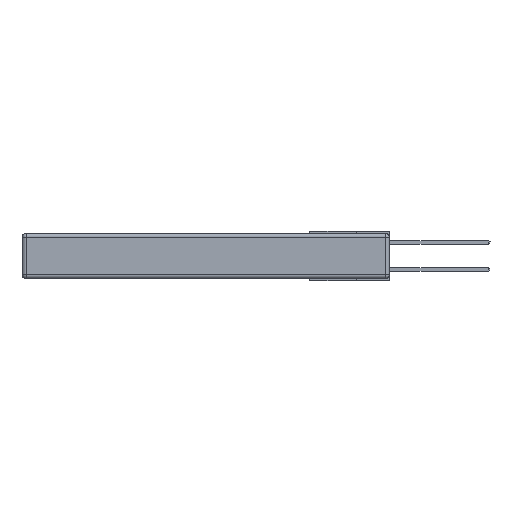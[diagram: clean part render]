
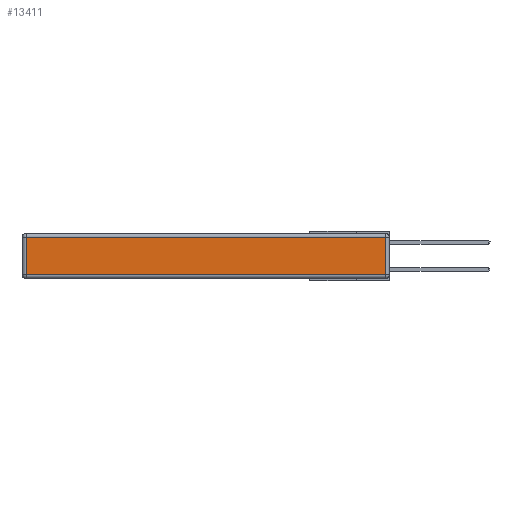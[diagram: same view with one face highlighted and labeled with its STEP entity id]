
A CAD part, left-side view. The second image highlights one B-rep face of the part: STEP entity #13411.
In plain terms, the highlighted planar face has unit normal (-1, 0, 0).
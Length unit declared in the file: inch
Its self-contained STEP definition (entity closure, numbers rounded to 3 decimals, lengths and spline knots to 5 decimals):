
#1149 = VERTEX_POINT ( 'NONE', #26603 ) ;
#1266 = CARTESIAN_POINT ( 'NONE',  ( 0., 2.75, -0.03 ) ) ;
#1762 = EDGE_LOOP ( 'NONE', ( #14225, #14690, #22841, #14623 ) ) ;
#2381 = VECTOR ( 'NONE', #23306, 39.37008 ) ;
#2400 = EDGE_CURVE ( 'NONE', #9237, #16036, #15914, .T. ) ;
#2862 = CARTESIAN_POINT ( 'NONE',  ( 0., 0.03, -0.343 ) ) ;
#3988 = EDGE_CURVE ( 'NONE', #16036, #24793, #28977, .T. ) ;
#4925 = DIRECTION ( 'NONE',  ( 0., 0., 1. ) ) ;
#7043 = PLANE ( 'NONE',  #23696 ) ;
#7703 = DIRECTION ( 'NONE',  ( 0., 1., 0. ) ) ;
#8486 = LINE ( 'NONE', #2862, #2381 ) ;
#9237 = VERTEX_POINT ( 'NONE', #14497 ) ;
#10323 = EDGE_CURVE ( 'NONE', #1149, #9237, #8486, .T. ) ;
#11277 = VECTOR ( 'NONE', #7703, 39.37008 ) ;
#13411 = ADVANCED_FACE ( 'NONE', ( #22712 ), #7043, .T. ) ;
#13749 = EDGE_CURVE ( 'NONE', #24793, #1149, #24820, .T. ) ;
#14225 = ORIENTED_EDGE ( 'NONE', *, *, #13749, .T. ) ;
#14497 = CARTESIAN_POINT ( 'NONE',  ( 0., 0.03, -0.03 ) ) ;
#14623 = ORIENTED_EDGE ( 'NONE', *, *, #3988, .T. ) ;
#14690 = ORIENTED_EDGE ( 'NONE', *, *, #10323, .T. ) ;
#14764 = CARTESIAN_POINT ( 'NONE',  ( 0., 0., -0.313 ) ) ;
#15914 = LINE ( 'NONE', #1266, #11277 ) ;
#16036 = VERTEX_POINT ( 'NONE', #29281 ) ;
#19340 = DIRECTION ( 'NONE',  ( 0., -1., 0. ) ) ;
#20223 = VECTOR ( 'NONE', #19340, 39.37008 ) ;
#20800 = VECTOR ( 'NONE', #28479, 39.37008 ) ;
#22712 = FACE_OUTER_BOUND ( 'NONE', #1762, .T. ) ;
#22773 = DIRECTION ( 'NONE',  ( -1., 0., 0. ) ) ;
#22841 = ORIENTED_EDGE ( 'NONE', *, *, #2400, .T. ) ;
#23056 = CARTESIAN_POINT ( 'NONE',  ( 0., 0., -0.343 ) ) ;
#23306 = DIRECTION ( 'NONE',  ( 0., 0., 1. ) ) ;
#23696 = AXIS2_PLACEMENT_3D ( 'NONE', #23056, #22773, #4925 ) ;
#24277 = CARTESIAN_POINT ( 'NONE',  ( 0., 2.72, -0.313 ) ) ;
#24793 = VERTEX_POINT ( 'NONE', #24277 ) ;
#24820 = LINE ( 'NONE', #14764, #20223 ) ;
#26171 = CARTESIAN_POINT ( 'NONE',  ( 0., 2.72, -0.343 ) ) ;
#26603 = CARTESIAN_POINT ( 'NONE',  ( 0., 0.03, -0.313 ) ) ;
#28479 = DIRECTION ( 'NONE',  ( 0., 0., -1. ) ) ;
#28977 = LINE ( 'NONE', #26171, #20800 ) ;
#29281 = CARTESIAN_POINT ( 'NONE',  ( 0., 2.72, -0.03 ) ) ;
